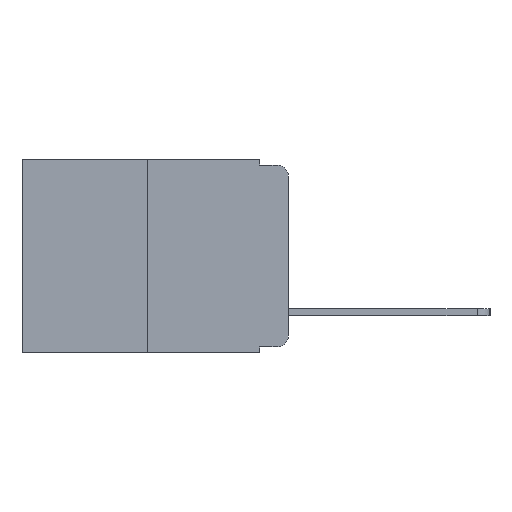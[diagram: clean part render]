
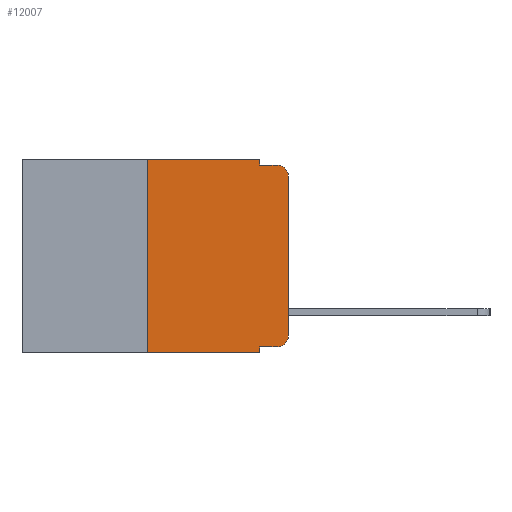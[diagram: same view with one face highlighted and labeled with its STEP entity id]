
A CAD part, left-side view. The second image highlights one B-rep face of the part: STEP entity #12007.
In plain terms, the highlighted planar face has unit normal (-1, 0, 0).
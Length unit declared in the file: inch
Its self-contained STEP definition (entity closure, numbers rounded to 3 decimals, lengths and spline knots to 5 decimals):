
#736 = ORIENTED_EDGE ( 'NONE', *, *, #18676, .T. ) ;
#874 = PLANE ( 'NONE',  #11292 ) ;
#1151 = CIRCLE ( 'NONE', #18702, 0.02 ) ;
#1800 = CIRCLE ( 'NONE', #24033, 0.02 ) ;
#2036 = CARTESIAN_POINT ( 'NONE',  ( 0., 0.051, 0. ) ) ;
#2881 = DIRECTION ( 'NONE',  ( 0., -1., 0. ) ) ;
#3190 = VECTOR ( 'NONE', #2881, 39.37008 ) ;
#3352 = EDGE_CURVE ( 'NONE', #14769, #9198, #15233, .T. ) ;
#3472 = VECTOR ( 'NONE', #7151, 39.37008 ) ;
#3893 = VERTEX_POINT ( 'NONE', #22787 ) ;
#3912 = DIRECTION ( 'NONE',  ( 0., -1., 0. ) ) ;
#4618 = VECTOR ( 'NONE', #3912, 39.37008 ) ;
#4746 = EDGE_CURVE ( 'NONE', #15909, #9198, #1800, .T. ) ;
#4903 = DIRECTION ( 'NONE',  ( -1., 0., 0. ) ) ;
#4937 = ORIENTED_EDGE ( 'NONE', *, *, #19994, .F. ) ;
#5885 = LINE ( 'NONE', #25735, #4618 ) ;
#6496 = ORIENTED_EDGE ( 'NONE', *, *, #7458, .T. ) ;
#6821 = VERTEX_POINT ( 'NONE', #18455 ) ;
#7151 = DIRECTION ( 'NONE',  ( 0., -1., 0. ) ) ;
#7458 = EDGE_CURVE ( 'NONE', #16026, #15909, #8395, .T. ) ;
#7616 = LINE ( 'NONE', #19145, #3472 ) ;
#7760 = ORIENTED_EDGE ( 'NONE', *, *, #13911, .F. ) ;
#7991 = CARTESIAN_POINT ( 'NONE',  ( 0., 0.02, -0.01 ) ) ;
#8208 = CARTESIAN_POINT ( 'NONE',  ( 0., 0.051, 0. ) ) ;
#8395 = LINE ( 'NONE', #20656, #23617 ) ;
#8580 = LINE ( 'NONE', #17002, #3190 ) ;
#9032 = ORIENTED_EDGE ( 'NONE', *, *, #13240, .T. ) ;
#9198 = VERTEX_POINT ( 'NONE', #7991 ) ;
#9591 = CARTESIAN_POINT ( 'NONE',  ( 0., 0., -0.313 ) ) ;
#9849 = CARTESIAN_POINT ( 'NONE',  ( 0., 0.02, -0.03 ) ) ;
#10043 = CARTESIAN_POINT ( 'NONE',  ( 0., 0.25, 0. ) ) ;
#10140 = DIRECTION ( 'NONE',  ( 0., 0., -1. ) ) ;
#11141 = DIRECTION ( 'NONE',  ( 1., 0., 0. ) ) ;
#11292 = AXIS2_PLACEMENT_3D ( 'NONE', #22954, #11141, #24904 ) ;
#11294 = VECTOR ( 'NONE', #10140, 39.37008 ) ;
#11881 = DIRECTION ( 'NONE',  ( 0., 0., -1. ) ) ;
#11887 = ORIENTED_EDGE ( 'NONE', *, *, #4746, .T. ) ;
#11929 = VERTEX_POINT ( 'NONE', #16872 ) ;
#12007 = ADVANCED_FACE ( 'NONE', ( #17924 ), #874, .F. ) ;
#12532 = ORIENTED_EDGE ( 'NONE', *, *, #3352, .F. ) ;
#12834 = EDGE_LOOP ( 'NONE', ( #6496, #11887, #12532, #23000, #7760, #19041, #9032, #4937, #736, #16870 ) ) ;
#13240 = EDGE_CURVE ( 'NONE', #17217, #20181, #8580, .T. ) ;
#13911 = EDGE_CURVE ( 'NONE', #17101, #11929, #7616, .T. ) ;
#14578 = VECTOR ( 'NONE', #19391, 39.37008 ) ;
#14769 = VERTEX_POINT ( 'NONE', #25036 ) ;
#15120 = LINE ( 'NONE', #17659, #24892 ) ;
#15233 = LINE ( 'NONE', #19397, #14578 ) ;
#15646 = VECTOR ( 'NONE', #24074, 39.37008 ) ;
#15909 = VERTEX_POINT ( 'NONE', #19124 ) ;
#16026 = VERTEX_POINT ( 'NONE', #9591 ) ;
#16270 = LINE ( 'NONE', #8208, #15646 ) ;
#16793 = DIRECTION ( 'NONE',  ( 0., 0., 1. ) ) ;
#16870 = ORIENTED_EDGE ( 'NONE', *, *, #17371, .T. ) ;
#16872 = CARTESIAN_POINT ( 'NONE',  ( 0., 0.051, 0. ) ) ;
#16928 = CARTESIAN_POINT ( 'NONE',  ( 0., 0.02, -0.313 ) ) ;
#17002 = CARTESIAN_POINT ( 'NONE',  ( 0., 0.473, -0.343 ) ) ;
#17101 = VERTEX_POINT ( 'NONE', #10043 ) ;
#17217 = VERTEX_POINT ( 'NONE', #18310 ) ;
#17371 = EDGE_CURVE ( 'NONE', #3893, #16026, #1151, .T. ) ;
#17659 = CARTESIAN_POINT ( 'NONE',  ( 0., 0.25, 0. ) ) ;
#17924 = FACE_OUTER_BOUND ( 'NONE', #12834, .T. ) ;
#18310 = CARTESIAN_POINT ( 'NONE',  ( 0., 0.25, -0.343 ) ) ;
#18455 = CARTESIAN_POINT ( 'NONE',  ( 0., 0.051, -0.333 ) ) ;
#18676 = EDGE_CURVE ( 'NONE', #6821, #3893, #5885, .T. ) ;
#18702 = AXIS2_PLACEMENT_3D ( 'NONE', #16928, #4903, #18922 ) ;
#18922 = DIRECTION ( 'NONE',  ( 0., 0., -1. ) ) ;
#19041 = ORIENTED_EDGE ( 'NONE', *, *, #23908, .F. ) ;
#19124 = CARTESIAN_POINT ( 'NONE',  ( 0., 0., -0.03 ) ) ;
#19145 = CARTESIAN_POINT ( 'NONE',  ( 0., 0.473, 0. ) ) ;
#19391 = DIRECTION ( 'NONE',  ( 0., -1., 0. ) ) ;
#19397 = CARTESIAN_POINT ( 'NONE',  ( 0., 0.051, -0.01 ) ) ;
#19627 = DIRECTION ( 'NONE',  ( 0., 0., 1. ) ) ;
#19994 = EDGE_CURVE ( 'NONE', #6821, #20181, #21801, .T. ) ;
#20181 = VERTEX_POINT ( 'NONE', #24545 ) ;
#20656 = CARTESIAN_POINT ( 'NONE',  ( 0., 0., 0. ) ) ;
#21801 = LINE ( 'NONE', #2036, #11294 ) ;
#22787 = CARTESIAN_POINT ( 'NONE',  ( 0., 0.02, -0.333 ) ) ;
#22954 = CARTESIAN_POINT ( 'NONE',  ( 0., 0.473, 0. ) ) ;
#23000 = ORIENTED_EDGE ( 'NONE', *, *, #25221, .F. ) ;
#23617 = VECTOR ( 'NONE', #16793, 39.37008 ) ;
#23678 = DIRECTION ( 'NONE',  ( -1., 0., 0. ) ) ;
#23908 = EDGE_CURVE ( 'NONE', #17217, #17101, #15120, .T. ) ;
#24033 = AXIS2_PLACEMENT_3D ( 'NONE', #9849, #23678, #11881 ) ;
#24074 = DIRECTION ( 'NONE',  ( 0., 0., -1. ) ) ;
#24545 = CARTESIAN_POINT ( 'NONE',  ( 0., 0.051, -0.343 ) ) ;
#24892 = VECTOR ( 'NONE', #19627, 39.37008 ) ;
#24904 = DIRECTION ( 'NONE',  ( 0., 0., -1. ) ) ;
#25036 = CARTESIAN_POINT ( 'NONE',  ( 0., 0.051, -0.01 ) ) ;
#25221 = EDGE_CURVE ( 'NONE', #11929, #14769, #16270, .T. ) ;
#25735 = CARTESIAN_POINT ( 'NONE',  ( 0., 0.051, -0.333 ) ) ;
